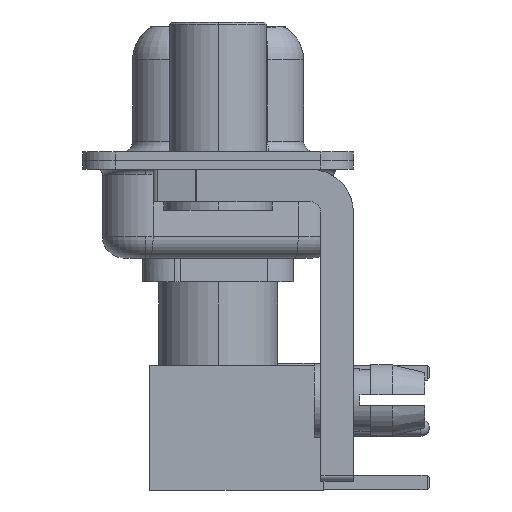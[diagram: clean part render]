
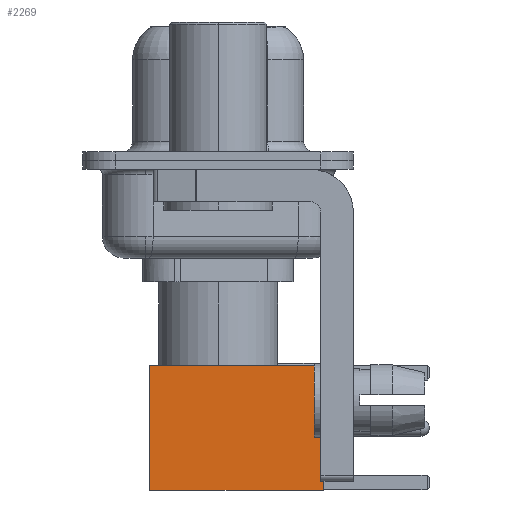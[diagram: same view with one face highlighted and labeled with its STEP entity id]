
A CAD part, left-side view. The second image highlights one B-rep face of the part: STEP entity #2269.
In plain terms, the highlighted face is planar.
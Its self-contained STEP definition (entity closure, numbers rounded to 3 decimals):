
#562 = LINE ( 'NONE', #10124, #1577 ) ;
#849 = CARTESIAN_POINT ( 'NONE',  ( 2.875, 2.875, 8. ) ) ;
#1577 = VECTOR ( 'NONE', #7929, 1000. ) ;
#2269 = ADVANCED_FACE ( 'NONE', ( #17046 ), #8085, .T. ) ;
#2362 = EDGE_CURVE ( 'NONE', #20691, #21170, #562, .T. ) ;
#5057 = CARTESIAN_POINT ( 'NONE',  ( -2.875, 2.875, 8. ) ) ;
#5074 = LINE ( 'NONE', #19507, #22229 ) ;
#5477 = VERTEX_POINT ( 'NONE', #11473 ) ;
#5578 = DIRECTION ( 'NONE',  ( 0., 0., 1. ) ) ;
#6419 = VERTEX_POINT ( 'NONE', #28202 ) ;
#7929 = DIRECTION ( 'NONE',  ( -1., 0., 0. ) ) ;
#8085 = PLANE ( 'NONE',  #21569 ) ;
#8124 = LINE ( 'NONE', #10320, #27872 ) ;
#8791 = EDGE_CURVE ( 'NONE', #6419, #5477, #16119, .T. ) ;
#10123 = EDGE_CURVE ( 'NONE', #20691, #6419, #8124, .T. ) ;
#10124 = CARTESIAN_POINT ( 'NONE',  ( 0., 2.875, 8. ) ) ;
#10320 = CARTESIAN_POINT ( 'NONE',  ( 2.875, 2.875, 0. ) ) ;
#11473 = CARTESIAN_POINT ( 'NONE',  ( -2.875, 2.875, 0. ) ) ;
#13921 = EDGE_CURVE ( 'NONE', #21170, #5477, #5074, .T. ) ;
#14238 = ORIENTED_EDGE ( 'NONE', *, *, #8791, .T. ) ;
#14637 = DIRECTION ( 'NONE',  ( 0., 0., -1. ) ) ;
#16119 = LINE ( 'NONE', #30270, #21341 ) ;
#17046 = FACE_OUTER_BOUND ( 'NONE', #26323, .T. ) ;
#18294 = ORIENTED_EDGE ( 'NONE', *, *, #2362, .F. ) ;
#19507 = CARTESIAN_POINT ( 'NONE',  ( -2.875, 2.875, 0. ) ) ;
#20000 = DIRECTION ( 'NONE',  ( 0., 1., 0. ) ) ;
#20691 = VERTEX_POINT ( 'NONE', #849 ) ;
#21170 = VERTEX_POINT ( 'NONE', #5057 ) ;
#21341 = VECTOR ( 'NONE', #25687, 1000. ) ;
#21569 = AXIS2_PLACEMENT_3D ( 'NONE', #26461, #20000, #5578 ) ;
#22229 = VECTOR ( 'NONE', #14637, 1000. ) ;
#24461 = DIRECTION ( 'NONE',  ( 0., 0., -1. ) ) ;
#25687 = DIRECTION ( 'NONE',  ( -1., 0., 0. ) ) ;
#26323 = EDGE_LOOP ( 'NONE', ( #30964, #14238, #29412, #18294 ) ) ;
#26461 = CARTESIAN_POINT ( 'NONE',  ( 2.875, 2.875, 0. ) ) ;
#27872 = VECTOR ( 'NONE', #24461, 1000. ) ;
#28202 = CARTESIAN_POINT ( 'NONE',  ( 2.875, 2.875, 0. ) ) ;
#29412 = ORIENTED_EDGE ( 'NONE', *, *, #13921, .F. ) ;
#30270 = CARTESIAN_POINT ( 'NONE',  ( 0., 2.875, 0. ) ) ;
#30964 = ORIENTED_EDGE ( 'NONE', *, *, #10123, .T. ) ;
